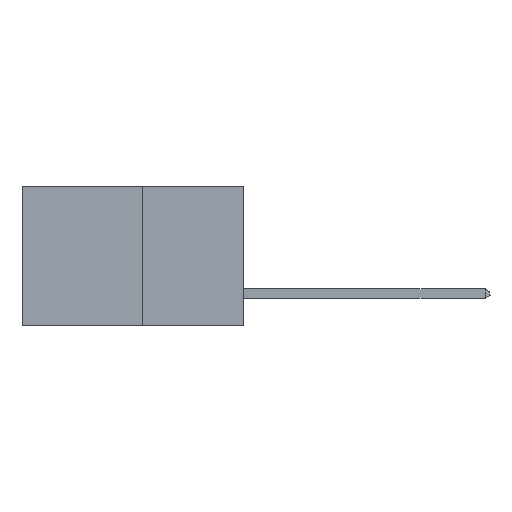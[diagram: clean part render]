
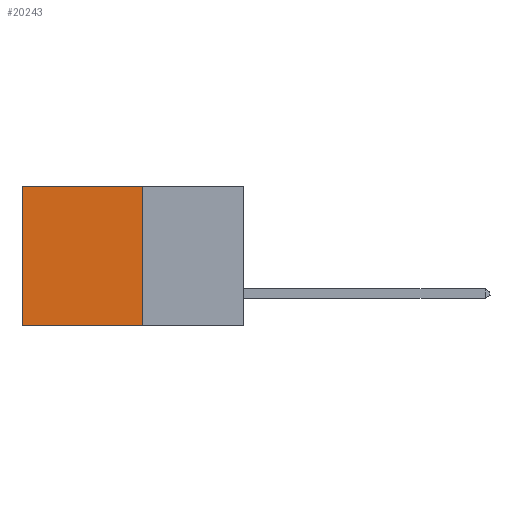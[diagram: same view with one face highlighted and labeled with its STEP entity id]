
A CAD part, left-side view. The second image highlights one B-rep face of the part: STEP entity #20243.
In plain terms, the highlighted planar face has unit normal (-1, 0, 0).
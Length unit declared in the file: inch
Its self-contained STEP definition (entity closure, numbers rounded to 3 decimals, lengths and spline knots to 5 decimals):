
#37 = PLANE ( 'NONE',  #12233 ) ;
#88 = FACE_OUTER_BOUND ( 'NONE', #10456, .T. ) ;
#1590 = ORIENTED_EDGE ( 'NONE', *, *, #4729, .T. ) ;
#1823 = DIRECTION ( 'NONE',  ( 0., 1., 0. ) ) ;
#1877 = DIRECTION ( 'NONE',  ( 0., 0., -1. ) ) ;
#1978 = DIRECTION ( 'NONE',  ( 0., 0., -1. ) ) ;
#3367 = LINE ( 'NONE', #22655, #16000 ) ;
#3382 = ORIENTED_EDGE ( 'NONE', *, *, #14042, .F. ) ;
#3549 = VECTOR ( 'NONE', #16947, 39.37008 ) ;
#3946 = VERTEX_POINT ( 'NONE', #22267 ) ;
#4425 = CARTESIAN_POINT ( 'NONE',  ( 0.277, 0.27, 0. ) ) ;
#4729 = EDGE_CURVE ( 'NONE', #10211, #8575, #3367, .T. ) ;
#5137 = ORIENTED_EDGE ( 'NONE', *, *, #21557, .F. ) ;
#5622 = CARTESIAN_POINT ( 'NONE',  ( 0.277, 0.27, -0.37 ) ) ;
#5630 = ORIENTED_EDGE ( 'NONE', *, *, #9120, .T. ) ;
#8575 = VERTEX_POINT ( 'NONE', #10170 ) ;
#8625 = LINE ( 'NONE', #12834, #13368 ) ;
#9120 = EDGE_CURVE ( 'NONE', #15238, #10211, #17291, .T. ) ;
#9713 = LINE ( 'NONE', #5622, #10773 ) ;
#10170 = CARTESIAN_POINT ( 'NONE',  ( 0.277, 0.59, -0.37 ) ) ;
#10211 = VERTEX_POINT ( 'NONE', #16368 ) ;
#10456 = EDGE_LOOP ( 'NONE', ( #1590, #3382, #5137, #5630 ) ) ;
#10773 = VECTOR ( 'NONE', #1823, 39.37008 ) ;
#12233 = AXIS2_PLACEMENT_3D ( 'NONE', #14472, #12730, #1877 ) ;
#12730 = DIRECTION ( 'NONE',  ( 1., 0., 0. ) ) ;
#12834 = CARTESIAN_POINT ( 'NONE',  ( 0.277, 0.27, -0.37 ) ) ;
#13368 = VECTOR ( 'NONE', #1978, 39.37008 ) ;
#14042 = EDGE_CURVE ( 'NONE', #3946, #8575, #9713, .T. ) ;
#14136 = CARTESIAN_POINT ( 'NONE',  ( 0.277, 0.27, 0. ) ) ;
#14472 = CARTESIAN_POINT ( 'NONE',  ( 0.277, 0.27, -0.37 ) ) ;
#15238 = VERTEX_POINT ( 'NONE', #14136 ) ;
#16000 = VECTOR ( 'NONE', #23039, 39.37008 ) ;
#16368 = CARTESIAN_POINT ( 'NONE',  ( 0.277, 0.59, 0. ) ) ;
#16947 = DIRECTION ( 'NONE',  ( 0., 1., 0. ) ) ;
#17291 = LINE ( 'NONE', #4425, #3549 ) ;
#20243 = ADVANCED_FACE ( 'NONE', ( #88 ), #37, .F. ) ;
#21557 = EDGE_CURVE ( 'NONE', #15238, #3946, #8625, .T. ) ;
#22267 = CARTESIAN_POINT ( 'NONE',  ( 0.277, 0.27, -0.37 ) ) ;
#22655 = CARTESIAN_POINT ( 'NONE',  ( 0.277, 0.59, -0.37 ) ) ;
#23039 = DIRECTION ( 'NONE',  ( 0., 0., -1. ) ) ;
